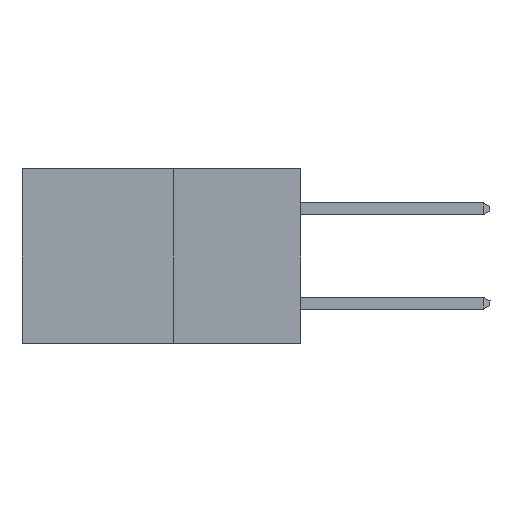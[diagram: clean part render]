
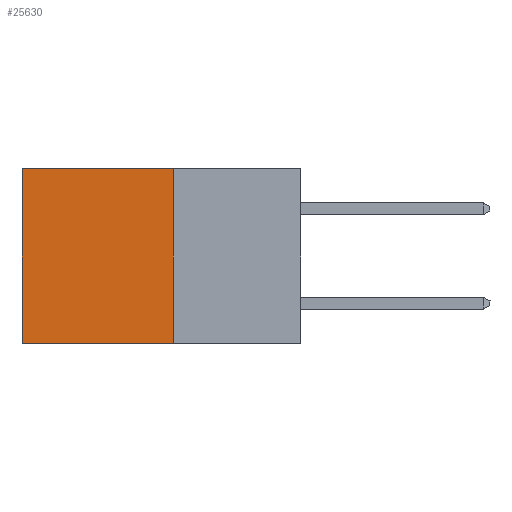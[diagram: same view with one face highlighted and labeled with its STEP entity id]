
A CAD part, left-side view. The second image highlights one B-rep face of the part: STEP entity #25630.
In plain terms, the highlighted planar face has unit normal (-1, 0, 0).
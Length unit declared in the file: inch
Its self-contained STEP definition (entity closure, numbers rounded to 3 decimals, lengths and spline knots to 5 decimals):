
#113 = VECTOR ( 'NONE', #2482, 39.37008 ) ;
#195 = DIRECTION ( 'NONE',  ( 0., 0., -1. ) ) ;
#573 = VERTEX_POINT ( 'NONE', #9449 ) ;
#2482 = DIRECTION ( 'NONE',  ( 0., 0., -1. ) ) ;
#2629 = VERTEX_POINT ( 'NONE', #20416 ) ;
#3528 = DIRECTION ( 'NONE',  ( 0., 1., 0. ) ) ;
#3569 = VECTOR ( 'NONE', #12241, 39.37008 ) ;
#4193 = VERTEX_POINT ( 'NONE', #24977 ) ;
#4220 = EDGE_LOOP ( 'NONE', ( #17358, #23265, #23956, #15640 ) ) ;
#6556 = VERTEX_POINT ( 'NONE', #16933 ) ;
#9210 = LINE ( 'NONE', #26681, #3569 ) ;
#9449 = CARTESIAN_POINT ( 'NONE',  ( 0.277, 0.27, 0. ) ) ;
#9956 = FACE_OUTER_BOUND ( 'NONE', #4220, .T. ) ;
#10635 = DIRECTION ( 'NONE',  ( 0., 0., -1. ) ) ;
#12006 = EDGE_CURVE ( 'NONE', #4193, #2629, #29236, .T. ) ;
#12216 = LINE ( 'NONE', #26596, #113 ) ;
#12235 = CARTESIAN_POINT ( 'NONE',  ( 0.277, 0.27, -0.37 ) ) ;
#12241 = DIRECTION ( 'NONE',  ( 0., 1., 0. ) ) ;
#13941 = LINE ( 'NONE', #12235, #25255 ) ;
#15477 = CARTESIAN_POINT ( 'NONE',  ( 0.277, 0.27, -0.37 ) ) ;
#15640 = ORIENTED_EDGE ( 'NONE', *, *, #17267, .T. ) ;
#16836 = AXIS2_PLACEMENT_3D ( 'NONE', #22628, #25020, #10635 ) ;
#16933 = CARTESIAN_POINT ( 'NONE',  ( 0.277, 0.59, 0. ) ) ;
#17267 = EDGE_CURVE ( 'NONE', #573, #6556, #9210, .T. ) ;
#17358 = ORIENTED_EDGE ( 'NONE', *, *, #30476, .T. ) ;
#20218 = PLANE ( 'NONE',  #16836 ) ;
#20416 = CARTESIAN_POINT ( 'NONE',  ( 0.277, 0.59, -0.37 ) ) ;
#20871 = EDGE_CURVE ( 'NONE', #573, #4193, #13941, .T. ) ;
#22628 = CARTESIAN_POINT ( 'NONE',  ( 0.277, 0.27, -0.37 ) ) ;
#23265 = ORIENTED_EDGE ( 'NONE', *, *, #12006, .F. ) ;
#23956 = ORIENTED_EDGE ( 'NONE', *, *, #20871, .F. ) ;
#24977 = CARTESIAN_POINT ( 'NONE',  ( 0.277, 0.27, -0.37 ) ) ;
#25020 = DIRECTION ( 'NONE',  ( 1., 0., 0. ) ) ;
#25255 = VECTOR ( 'NONE', #195, 39.37008 ) ;
#25630 = ADVANCED_FACE ( 'NONE', ( #9956 ), #20218, .F. ) ;
#26596 = CARTESIAN_POINT ( 'NONE',  ( 0.277, 0.59, -0.37 ) ) ;
#26681 = CARTESIAN_POINT ( 'NONE',  ( 0.277, 0.27, 0. ) ) ;
#29236 = LINE ( 'NONE', #15477, #29975 ) ;
#29975 = VECTOR ( 'NONE', #3528, 39.37008 ) ;
#30476 = EDGE_CURVE ( 'NONE', #6556, #2629, #12216, .T. ) ;
